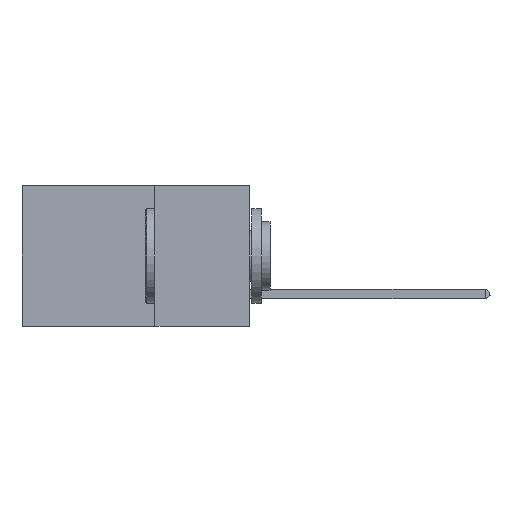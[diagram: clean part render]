
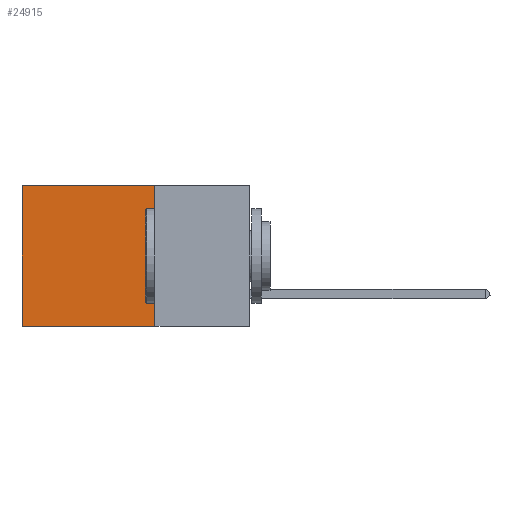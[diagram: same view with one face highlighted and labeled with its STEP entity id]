
A CAD part, left-side view. The second image highlights one B-rep face of the part: STEP entity #24915.
In plain terms, the highlighted planar face has unit normal (-1, 0, 0).
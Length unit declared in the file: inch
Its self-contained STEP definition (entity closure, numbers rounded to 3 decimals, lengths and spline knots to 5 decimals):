
#365 = ORIENTED_EDGE ( 'NONE', *, *, #40972, .F. ) ;
#1197 = VERTEX_POINT ( 'NONE', #5036 ) ;
#1602 = VECTOR ( 'NONE', #3520, 39.37008 ) ;
#3520 = DIRECTION ( 'NONE',  ( 0., 1., 0. ) ) ;
#3739 = DIRECTION ( 'NONE',  ( 0., 0., -1. ) ) ;
#5036 = CARTESIAN_POINT ( 'NONE',  ( 0.2875, 0.6, -0.37 ) ) ;
#5261 = EDGE_LOOP ( 'NONE', ( #15910, #31116, #365, #25156 ) ) ;
#5589 = CARTESIAN_POINT ( 'NONE',  ( 0.2875, 0.25, 0. ) ) ;
#8250 = VERTEX_POINT ( 'NONE', #18537 ) ;
#9538 = LINE ( 'NONE', #37069, #42473 ) ;
#10162 = AXIS2_PLACEMENT_3D ( 'NONE', #26766, #46225, #13018 ) ;
#10447 = LINE ( 'NONE', #26790, #25226 ) ;
#13018 = DIRECTION ( 'NONE',  ( 0., 0., -1. ) ) ;
#15396 = VERTEX_POINT ( 'NONE', #24068 ) ;
#15910 = ORIENTED_EDGE ( 'NONE', *, *, #44141, .T. ) ;
#18537 = CARTESIAN_POINT ( 'NONE',  ( 0.2875, 0.25, -0.37 ) ) ;
#18676 = LINE ( 'NONE', #25337, #1602 ) ;
#24068 = CARTESIAN_POINT ( 'NONE',  ( 0.2875, 0.6, 0. ) ) ;
#24915 = ADVANCED_FACE ( 'NONE', ( #26309 ), #30925, .F. ) ;
#25156 = ORIENTED_EDGE ( 'NONE', *, *, #34919, .T. ) ;
#25226 = VECTOR ( 'NONE', #44943, 39.37008 ) ;
#25337 = CARTESIAN_POINT ( 'NONE',  ( 0.2875, 0.25, 0. ) ) ;
#26309 = FACE_OUTER_BOUND ( 'NONE', #5261, .T. ) ;
#26766 = CARTESIAN_POINT ( 'NONE',  ( 0.2875, 0.25, 0. ) ) ;
#26790 = CARTESIAN_POINT ( 'NONE',  ( 0.2875, 0.25, 0. ) ) ;
#30925 = PLANE ( 'NONE',  #10162 ) ;
#31116 = ORIENTED_EDGE ( 'NONE', *, *, #46217, .F. ) ;
#34919 = EDGE_CURVE ( 'NONE', #40376, #15396, #18676, .T. ) ;
#36445 = CARTESIAN_POINT ( 'NONE',  ( 0.2875, 0.25, -0.37 ) ) ;
#37069 = CARTESIAN_POINT ( 'NONE',  ( 0.2875, 0.6, 0. ) ) ;
#37576 = VECTOR ( 'NONE', #40107, 39.37008 ) ;
#39377 = LINE ( 'NONE', #36445, #37576 ) ;
#40107 = DIRECTION ( 'NONE',  ( 0., 1., 0. ) ) ;
#40376 = VERTEX_POINT ( 'NONE', #5589 ) ;
#40972 = EDGE_CURVE ( 'NONE', #40376, #8250, #10447, .T. ) ;
#42473 = VECTOR ( 'NONE', #3739, 39.37008 ) ;
#44141 = EDGE_CURVE ( 'NONE', #15396, #1197, #9538, .T. ) ;
#44943 = DIRECTION ( 'NONE',  ( 0., 0., -1. ) ) ;
#46217 = EDGE_CURVE ( 'NONE', #8250, #1197, #39377, .T. ) ;
#46225 = DIRECTION ( 'NONE',  ( 1., 0., 0. ) ) ;
